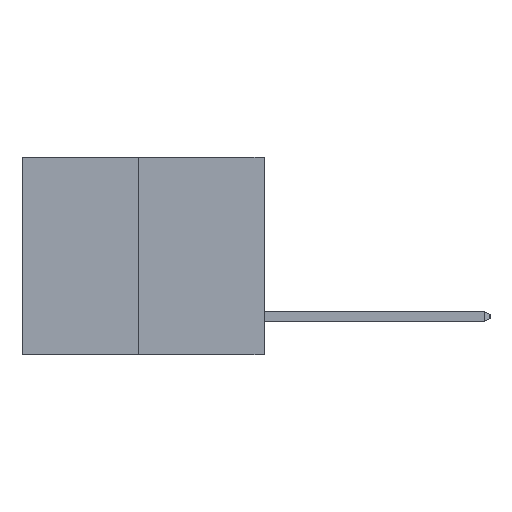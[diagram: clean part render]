
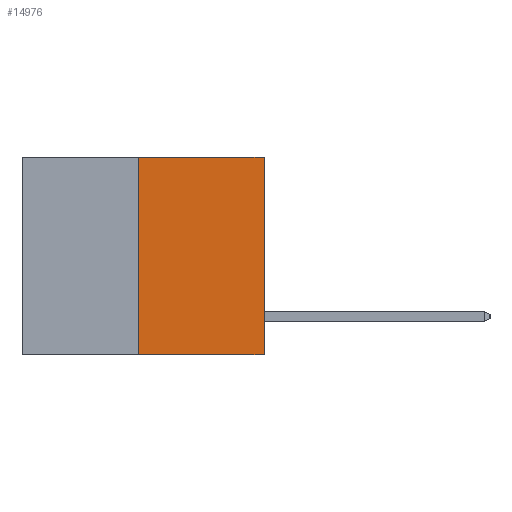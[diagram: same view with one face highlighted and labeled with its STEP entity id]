
A CAD part, left-side view. The second image highlights one B-rep face of the part: STEP entity #14976.
In plain terms, the highlighted planar face has unit normal (-1, 0, 0).
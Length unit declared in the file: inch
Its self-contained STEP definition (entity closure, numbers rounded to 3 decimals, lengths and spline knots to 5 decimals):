
#487 = VERTEX_POINT ( 'NONE', #21960 ) ;
#719 = EDGE_CURVE ( 'NONE', #13975, #487, #9584, .T. ) ;
#1095 = CARTESIAN_POINT ( 'NONE',  ( 0., 0., 0. ) ) ;
#1100 = CARTESIAN_POINT ( 'NONE',  ( 0., 0.6, 0. ) ) ;
#1243 = EDGE_CURVE ( 'NONE', #23857, #487, #13465, .T. ) ;
#1261 = DIRECTION ( 'NONE',  ( 0., 0., 1. ) ) ;
#2350 = LINE ( 'NONE', #4598, #18028 ) ;
#3436 = CARTESIAN_POINT ( 'NONE',  ( 0., 0.6, 0. ) ) ;
#3566 = VERTEX_POINT ( 'NONE', #14635 ) ;
#3792 = CARTESIAN_POINT ( 'NONE',  ( 0., 0., -0.49 ) ) ;
#4598 = CARTESIAN_POINT ( 'NONE',  ( 0., 0.312, -0.49 ) ) ;
#4767 = DIRECTION ( 'NONE',  ( 0., 0., 1. ) ) ;
#5240 = ORIENTED_EDGE ( 'NONE', *, *, #19748, .T. ) ;
#6004 = LINE ( 'NONE', #14652, #18017 ) ;
#7197 = EDGE_CURVE ( 'NONE', #3566, #13975, #2350, .T. ) ;
#7418 = CARTESIAN_POINT ( 'NONE',  ( 0., 0.312, 0. ) ) ;
#7572 = FACE_OUTER_BOUND ( 'NONE', #15465, .T. ) ;
#8954 = ORIENTED_EDGE ( 'NONE', *, *, #719, .F. ) ;
#9584 = LINE ( 'NONE', #3436, #19198 ) ;
#12142 = DIRECTION ( 'NONE',  ( 1., 0., 0. ) ) ;
#13465 = LINE ( 'NONE', #1095, #23626 ) ;
#13975 = VERTEX_POINT ( 'NONE', #7418 ) ;
#14635 = CARTESIAN_POINT ( 'NONE',  ( 0., 0.312, -0.49 ) ) ;
#14652 = CARTESIAN_POINT ( 'NONE',  ( 0., 0.6, -0.49 ) ) ;
#14976 = ADVANCED_FACE ( 'NONE', ( #7572 ), #18590, .F. ) ;
#15465 = EDGE_LOOP ( 'NONE', ( #23356, #5240, #17488, #8954 ) ) ;
#17488 = ORIENTED_EDGE ( 'NONE', *, *, #1243, .T. ) ;
#18017 = VECTOR ( 'NONE', #20945, 39.37008 ) ;
#18028 = VECTOR ( 'NONE', #4767, 39.37008 ) ;
#18590 = PLANE ( 'NONE',  #19040 ) ;
#19040 = AXIS2_PLACEMENT_3D ( 'NONE', #1100, #12142, #24284 ) ;
#19198 = VECTOR ( 'NONE', #22786, 39.37008 ) ;
#19748 = EDGE_CURVE ( 'NONE', #3566, #23857, #6004, .T. ) ;
#20945 = DIRECTION ( 'NONE',  ( 0., -1., 0. ) ) ;
#21960 = CARTESIAN_POINT ( 'NONE',  ( 0., 0., 0. ) ) ;
#22786 = DIRECTION ( 'NONE',  ( 0., -1., 0. ) ) ;
#23356 = ORIENTED_EDGE ( 'NONE', *, *, #7197, .F. ) ;
#23626 = VECTOR ( 'NONE', #1261, 39.37008 ) ;
#23857 = VERTEX_POINT ( 'NONE', #3792 ) ;
#24284 = DIRECTION ( 'NONE',  ( 0., 0., -1. ) ) ;
